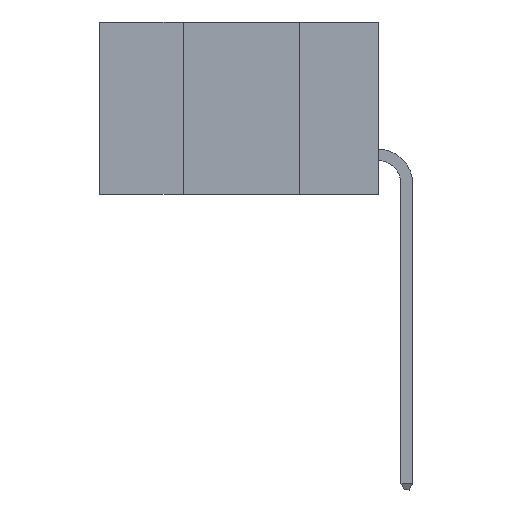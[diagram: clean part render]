
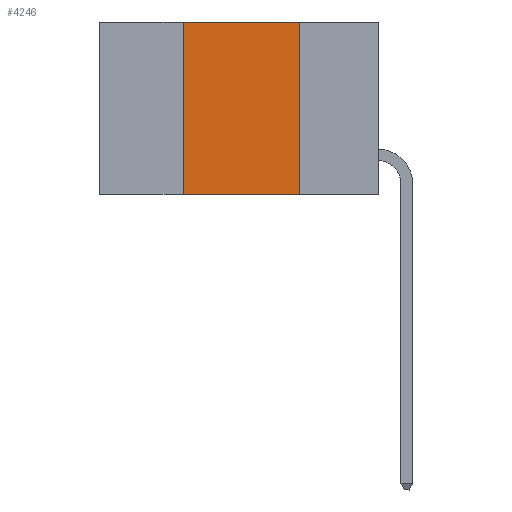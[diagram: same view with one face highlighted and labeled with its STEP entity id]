
A CAD part, left-side view. The second image highlights one B-rep face of the part: STEP entity #4246.
In plain terms, the highlighted planar face has unit normal (-1, 0, 0).
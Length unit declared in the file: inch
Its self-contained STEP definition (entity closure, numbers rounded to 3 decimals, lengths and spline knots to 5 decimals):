
#1 = CARTESIAN_POINT ( 'NONE',  ( 0., 0.6, 0. ) ) ;
#108 = DIRECTION ( 'NONE',  ( 0., -1., 0. ) ) ;
#130 = DIRECTION ( 'NONE',  ( 0., 0., -1. ) ) ;
#257 = DIRECTION ( 'NONE',  ( 0., -1., 0. ) ) ;
#467 = DIRECTION ( 'NONE',  ( 0., 0., 1. ) ) ;
#1007 = EDGE_CURVE ( 'NONE', #1357, #1613, #8113, .T. ) ;
#1357 = VERTEX_POINT ( 'NONE', #8666 ) ;
#1613 = VERTEX_POINT ( 'NONE', #7971 ) ;
#1639 = VECTOR ( 'NONE', #257, 39.37008 ) ;
#2076 = PLANE ( 'NONE',  #6821 ) ;
#2370 = EDGE_CURVE ( 'NONE', #1357, #10868, #8079, .T. ) ;
#3033 = FACE_OUTER_BOUND ( 'NONE', #7090, .T. ) ;
#3221 = VERTEX_POINT ( 'NONE', #5440 ) ;
#3691 = EDGE_CURVE ( 'NONE', #10868, #3221, #9373, .T. ) ;
#3839 = ORIENTED_EDGE ( 'NONE', *, *, #3691, .F. ) ;
#3972 = ORIENTED_EDGE ( 'NONE', *, *, #2370, .F. ) ;
#4057 = DIRECTION ( 'NONE',  ( 0., 0., -1. ) ) ;
#4246 = ADVANCED_FACE ( 'NONE', ( #3033 ), #2076, .F. ) ;
#4331 = LINE ( 'NONE', #10747, #8837 ) ;
#4874 = CARTESIAN_POINT ( 'NONE',  ( 0., 0.42, 0. ) ) ;
#4983 = EDGE_CURVE ( 'NONE', #3221, #1613, #4331, .T. ) ;
#5018 = ORIENTED_EDGE ( 'NONE', *, *, #4983, .F. ) ;
#5440 = CARTESIAN_POINT ( 'NONE',  ( 0., 0.17, 0. ) ) ;
#5522 = VECTOR ( 'NONE', #467, 39.37008 ) ;
#5836 = VECTOR ( 'NONE', #108, 39.37008 ) ;
#6328 = CARTESIAN_POINT ( 'NONE',  ( 0., 0.42, 0. ) ) ;
#6821 = AXIS2_PLACEMENT_3D ( 'NONE', #1, #9787, #4057 ) ;
#7090 = EDGE_LOOP ( 'NONE', ( #5018, #3839, #3972, #11738 ) ) ;
#7971 = CARTESIAN_POINT ( 'NONE',  ( 0., 0.17, -0.37 ) ) ;
#8079 = LINE ( 'NONE', #6328, #5522 ) ;
#8113 = LINE ( 'NONE', #11391, #5836 ) ;
#8666 = CARTESIAN_POINT ( 'NONE',  ( 0., 0.42, -0.37 ) ) ;
#8837 = VECTOR ( 'NONE', #130, 39.37008 ) ;
#9373 = LINE ( 'NONE', #11741, #1639 ) ;
#9787 = DIRECTION ( 'NONE',  ( 1., 0., 0. ) ) ;
#10747 = CARTESIAN_POINT ( 'NONE',  ( 0., 0.17, 0. ) ) ;
#10868 = VERTEX_POINT ( 'NONE', #4874 ) ;
#11391 = CARTESIAN_POINT ( 'NONE',  ( 0., 0.6, -0.37 ) ) ;
#11738 = ORIENTED_EDGE ( 'NONE', *, *, #1007, .T. ) ;
#11741 = CARTESIAN_POINT ( 'NONE',  ( 0., 0.6, 0. ) ) ;
